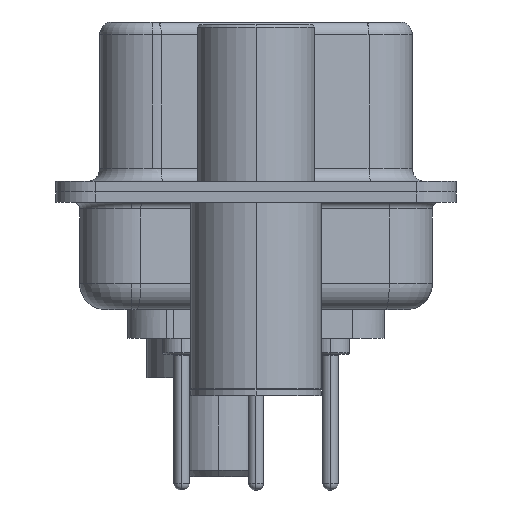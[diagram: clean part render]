
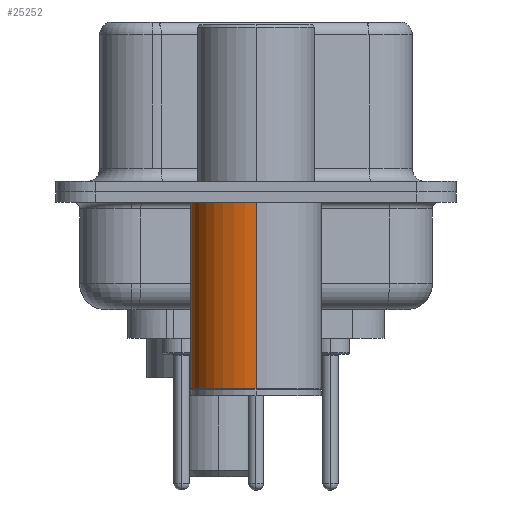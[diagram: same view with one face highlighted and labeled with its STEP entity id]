
A CAD part, left-side view. The second image highlights one B-rep face of the part: STEP entity #25252.
In plain terms, the highlighted cylindrical face has radius 2.5 mm (diameter 5 mm), a partial arc.
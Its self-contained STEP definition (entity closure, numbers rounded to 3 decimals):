
#892 = CARTESIAN_POINT ( 'NONE',  ( 0., 0., -7.525 ) ) ;
#908 = ORIENTED_EDGE ( 'NONE', *, *, #14690, .F. ) ;
#1574 = AXIS2_PLACEMENT_3D ( 'NONE', #892, #20452, #3451 ) ;
#1779 = ORIENTED_EDGE ( 'NONE', *, *, #10444, .F. ) ;
#2363 = AXIS2_PLACEMENT_3D ( 'NONE', #25713, #3042, #8743 ) ;
#2901 = VECTOR ( 'NONE', #16195, 1000. ) ;
#3042 = DIRECTION ( 'NONE',  ( 0., 0., 1. ) ) ;
#3363 = EDGE_CURVE ( 'NONE', #35304, #10216, #15704, .T. ) ;
#3451 = DIRECTION ( 'NONE',  ( 1., 0., 0. ) ) ;
#4904 = CARTESIAN_POINT ( 'NONE',  ( 2.5, 0., 0.581 ) ) ;
#5768 = CARTESIAN_POINT ( 'NONE',  ( 0., 0., -0.4 ) ) ;
#6783 = CARTESIAN_POINT ( 'NONE',  ( -2.5, 0., -0.4 ) ) ;
#8612 = DIRECTION ( 'NONE',  ( 1., 0., 0. ) ) ;
#8743 = DIRECTION ( 'NONE',  ( 1., 0., 0. ) ) ;
#10216 = VERTEX_POINT ( 'NONE', #12495 ) ;
#10323 = DIRECTION ( 'NONE',  ( 0., 0., 1. ) ) ;
#10444 = EDGE_CURVE ( 'NONE', #35304, #33915, #25521, .T. ) ;
#10707 = CARTESIAN_POINT ( 'NONE',  ( 2.5, 0., -0.4 ) ) ;
#12495 = CARTESIAN_POINT ( 'NONE',  ( -2.5, 0., -7.525 ) ) ;
#14690 = EDGE_CURVE ( 'NONE', #33915, #21648, #33557, .T. ) ;
#15120 = EDGE_CURVE ( 'NONE', #10216, #21648, #23041, .T. ) ;
#15526 = VECTOR ( 'NONE', #10323, 1000. ) ;
#15704 = CIRCLE ( 'NONE', #1574, 2.5 ) ;
#16195 = DIRECTION ( 'NONE',  ( 0., 0., 1. ) ) ;
#18643 = AXIS2_PLACEMENT_3D ( 'NONE', #5768, #25579, #8612 ) ;
#18724 = ORIENTED_EDGE ( 'NONE', *, *, #15120, .T. ) ;
#19817 = CYLINDRICAL_SURFACE ( 'NONE', #2363, 2.5 ) ;
#20452 = DIRECTION ( 'NONE',  ( 0., 0., 1. ) ) ;
#21648 = VERTEX_POINT ( 'NONE', #6783 ) ;
#23005 = ORIENTED_EDGE ( 'NONE', *, *, #3363, .T. ) ;
#23041 = LINE ( 'NONE', #24457, #15526 ) ;
#24457 = CARTESIAN_POINT ( 'NONE',  ( -2.5, 0., 0.581 ) ) ;
#25252 = ADVANCED_FACE ( 'NONE', ( #34700 ), #19817, .T. ) ;
#25521 = LINE ( 'NONE', #4904, #2901 ) ;
#25579 = DIRECTION ( 'NONE',  ( 0., 0., 1. ) ) ;
#25713 = CARTESIAN_POINT ( 'NONE',  ( 0., 0., 0.581 ) ) ;
#26134 = CARTESIAN_POINT ( 'NONE',  ( 2.5, 0., -7.525 ) ) ;
#29114 = EDGE_LOOP ( 'NONE', ( #23005, #18724, #908, #1779 ) ) ;
#33557 = CIRCLE ( 'NONE', #18643, 2.5 ) ;
#33915 = VERTEX_POINT ( 'NONE', #10707 ) ;
#34700 = FACE_OUTER_BOUND ( 'NONE', #29114, .T. ) ;
#35304 = VERTEX_POINT ( 'NONE', #26134 ) ;
